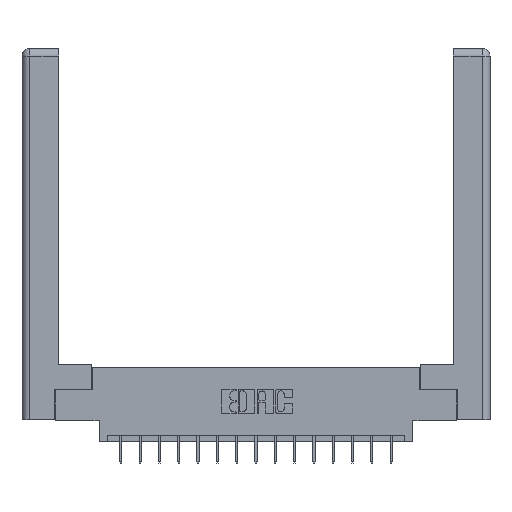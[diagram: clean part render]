
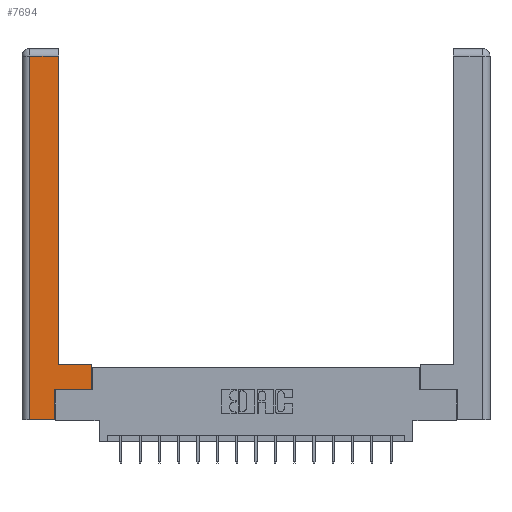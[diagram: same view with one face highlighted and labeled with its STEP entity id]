
A CAD part, top view. The second image highlights one B-rep face of the part: STEP entity #7694.
In plain terms, the highlighted planar face has unit normal (0, 0, 1).
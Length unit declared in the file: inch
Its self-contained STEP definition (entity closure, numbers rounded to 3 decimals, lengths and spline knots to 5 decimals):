
#453 = VECTOR ( 'NONE', #2751, 39.37008 ) ;
#551 = DIRECTION ( 'NONE',  ( -1., 0., 0. ) ) ;
#689 = LINE ( 'NONE', #14566, #12188 ) ;
#1124 = ORIENTED_EDGE ( 'NONE', *, *, #7701, .T. ) ;
#1237 = LINE ( 'NONE', #13097, #15138 ) ;
#1393 = ORIENTED_EDGE ( 'NONE', *, *, #9360, .T. ) ;
#1476 = VECTOR ( 'NONE', #5170, 39.37008 ) ;
#2109 = DIRECTION ( 'NONE',  ( 0., 0., -1. ) ) ;
#2568 = CARTESIAN_POINT ( 'NONE',  ( 0.0615, 0., 0. ) ) ;
#2751 = DIRECTION ( 'NONE',  ( 0., -1., 0. ) ) ;
#2806 = EDGE_CURVE ( 'NONE', #3531, #14899, #17026, .T. ) ;
#3003 = LINE ( 'NONE', #13487, #1476 ) ;
#3293 = DIRECTION ( 'NONE',  ( 1., 0., 0. ) ) ;
#3531 = VERTEX_POINT ( 'NONE', #11600 ) ;
#3574 = ORIENTED_EDGE ( 'NONE', *, *, #8594, .T. ) ;
#3735 = AXIS2_PLACEMENT_3D ( 'NONE', #11599, #2109, #551 ) ;
#3772 = DIRECTION ( 'NONE',  ( -1., 0., 0. ) ) ;
#3898 = VECTOR ( 'NONE', #3772, 39.37008 ) ;
#4055 = VERTEX_POINT ( 'NONE', #4512 ) ;
#4221 = VERTEX_POINT ( 'NONE', #15925 ) ;
#4512 = CARTESIAN_POINT ( 'NONE',  ( 0.295, 0.45, 0. ) ) ;
#5170 = DIRECTION ( 'NONE',  ( 0., 1., 0. ) ) ;
#5176 = VECTOR ( 'NONE', #3293, 39.37008 ) ;
#5235 = EDGE_LOOP ( 'NONE', ( #11807, #9813, #1393, #13859, #9743, #14122, #3574, #1124 ) ) ;
#5454 = CARTESIAN_POINT ( 'NONE',  ( 0.565, 0.45, 0. ) ) ;
#5912 = EDGE_CURVE ( 'NONE', #12050, #11446, #6542, .T. ) ;
#6181 = DIRECTION ( 'NONE',  ( -1., 0., 0. ) ) ;
#6529 = CARTESIAN_POINT ( 'NONE',  ( 0.0615, 2.94, 0. ) ) ;
#6542 = LINE ( 'NONE', #16995, #3898 ) ;
#7002 = LINE ( 'NONE', #2568, #453 ) ;
#7688 = DIRECTION ( 'NONE',  ( 1., 0., 0. ) ) ;
#7694 = ADVANCED_FACE ( 'NONE', ( #10721 ), #16948, .F. ) ;
#7701 = EDGE_CURVE ( 'NONE', #10768, #4055, #10120, .T. ) ;
#8000 = CARTESIAN_POINT ( 'NONE',  ( 0.265, 0.245, 0. ) ) ;
#8594 = EDGE_CURVE ( 'NONE', #13560, #10768, #689, .T. ) ;
#9360 = EDGE_CURVE ( 'NONE', #11446, #4221, #7002, .T. ) ;
#9667 = VECTOR ( 'NONE', #17209, 39.37008 ) ;
#9743 = ORIENTED_EDGE ( 'NONE', *, *, #2806, .T. ) ;
#9813 = ORIENTED_EDGE ( 'NONE', *, *, #5912, .T. ) ;
#10120 = LINE ( 'NONE', #14526, #16789 ) ;
#10297 = CARTESIAN_POINT ( 'NONE',  ( 0.265, 0., 0. ) ) ;
#10721 = FACE_OUTER_BOUND ( 'NONE', #5235, .T. ) ;
#10768 = VERTEX_POINT ( 'NONE', #5454 ) ;
#11446 = VERTEX_POINT ( 'NONE', #6529 ) ;
#11506 = CARTESIAN_POINT ( 'NONE',  ( 0.265, 0.245, 0. ) ) ;
#11599 = CARTESIAN_POINT ( 'NONE',  ( 0., 0., 0. ) ) ;
#11600 = CARTESIAN_POINT ( 'NONE',  ( 0.265, 0., 0. ) ) ;
#11807 = ORIENTED_EDGE ( 'NONE', *, *, #16101, .T. ) ;
#11993 = CARTESIAN_POINT ( 'NONE',  ( 0.295, 2.94, 0. ) ) ;
#12050 = VERTEX_POINT ( 'NONE', #11993 ) ;
#12093 = LINE ( 'NONE', #10297, #5176 ) ;
#12188 = VECTOR ( 'NONE', #12276, 39.37008 ) ;
#12276 = DIRECTION ( 'NONE',  ( 0., 1., 0. ) ) ;
#13097 = CARTESIAN_POINT ( 'NONE',  ( 0.565, 0.245, 0. ) ) ;
#13487 = CARTESIAN_POINT ( 'NONE',  ( 0.295, 3., 0. ) ) ;
#13560 = VERTEX_POINT ( 'NONE', #15420 ) ;
#13859 = ORIENTED_EDGE ( 'NONE', *, *, #16566, .T. ) ;
#14122 = ORIENTED_EDGE ( 'NONE', *, *, #17315, .T. ) ;
#14526 = CARTESIAN_POINT ( 'NONE',  ( 0.295, 0.45, 0. ) ) ;
#14566 = CARTESIAN_POINT ( 'NONE',  ( 0.565, 0.45, 0. ) ) ;
#14899 = VERTEX_POINT ( 'NONE', #8000 ) ;
#15138 = VECTOR ( 'NONE', #7688, 39.37008 ) ;
#15420 = CARTESIAN_POINT ( 'NONE',  ( 0.565, 0.245, 0. ) ) ;
#15925 = CARTESIAN_POINT ( 'NONE',  ( 0.0615, 0., 0. ) ) ;
#16101 = EDGE_CURVE ( 'NONE', #4055, #12050, #3003, .T. ) ;
#16566 = EDGE_CURVE ( 'NONE', #4221, #3531, #12093, .T. ) ;
#16789 = VECTOR ( 'NONE', #6181, 39.37008 ) ;
#16948 = PLANE ( 'NONE',  #3735 ) ;
#16995 = CARTESIAN_POINT ( 'NONE',  ( 0.0615, 2.94, 0. ) ) ;
#17026 = LINE ( 'NONE', #11506, #9667 ) ;
#17209 = DIRECTION ( 'NONE',  ( 0., 1., 0. ) ) ;
#17315 = EDGE_CURVE ( 'NONE', #14899, #13560, #1237, .T. ) ;
